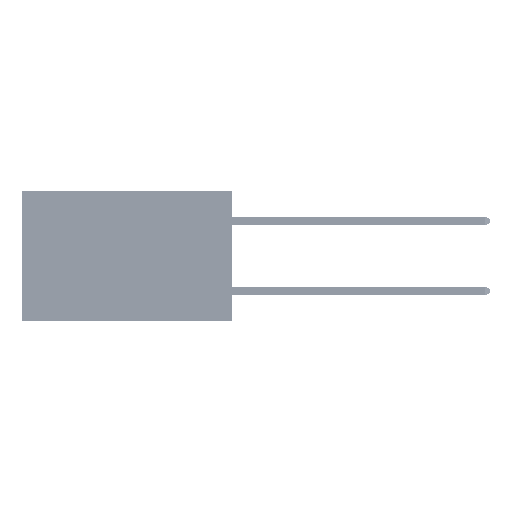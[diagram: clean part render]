
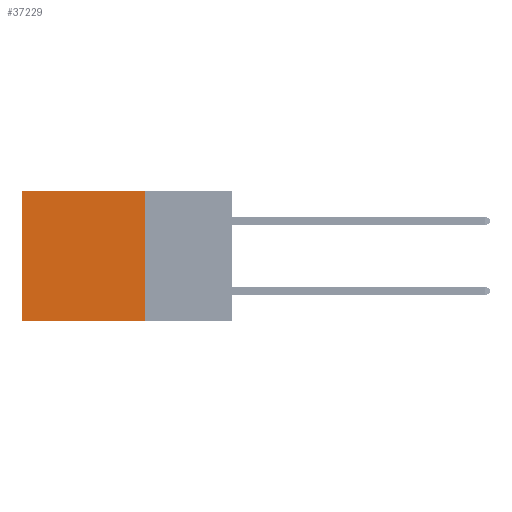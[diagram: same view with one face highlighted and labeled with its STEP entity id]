
A CAD part, left-side view. The second image highlights one B-rep face of the part: STEP entity #37229.
In plain terms, the highlighted planar face has unit normal (-1, 0, 0).
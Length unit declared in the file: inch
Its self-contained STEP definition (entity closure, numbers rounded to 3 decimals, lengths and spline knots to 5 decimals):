
#192 = CARTESIAN_POINT ( 'NONE',  ( 0.2875, 0.25, 0. ) ) ;
#3415 = VECTOR ( 'NONE', #33637, 39.37008 ) ;
#3467 = EDGE_CURVE ( 'NONE', #28301, #17805, #35521, .T. ) ;
#4042 = ORIENTED_EDGE ( 'NONE', *, *, #40278, .T. ) ;
#5532 = CARTESIAN_POINT ( 'NONE',  ( 0.2875, 0.25, -0.37 ) ) ;
#6696 = VERTEX_POINT ( 'NONE', #23124 ) ;
#11294 = VECTOR ( 'NONE', #22963, 39.37008 ) ;
#14636 = EDGE_CURVE ( 'NONE', #6696, #17805, #23315, .T. ) ;
#15011 = LINE ( 'NONE', #192, #49844 ) ;
#15630 = CARTESIAN_POINT ( 'NONE',  ( 0.2875, 0.25, 0. ) ) ;
#17805 = VERTEX_POINT ( 'NONE', #40143 ) ;
#22963 = DIRECTION ( 'NONE',  ( 0., 0., -1. ) ) ;
#23124 = CARTESIAN_POINT ( 'NONE',  ( 0.2875, 0.6, 0. ) ) ;
#23315 = LINE ( 'NONE', #30748, #11294 ) ;
#25441 = EDGE_LOOP ( 'NONE', ( #36223, #34992, #48789, #4042 ) ) ;
#28301 = VERTEX_POINT ( 'NONE', #50284 ) ;
#30748 = CARTESIAN_POINT ( 'NONE',  ( 0.2875, 0.6, 0. ) ) ;
#33637 = DIRECTION ( 'NONE',  ( 0., 1., 0. ) ) ;
#34992 = ORIENTED_EDGE ( 'NONE', *, *, #3467, .F. ) ;
#35521 = LINE ( 'NONE', #5532, #3415 ) ;
#36223 = ORIENTED_EDGE ( 'NONE', *, *, #14636, .T. ) ;
#36271 = DIRECTION ( 'NONE',  ( 0., 0., -1. ) ) ;
#37229 = ADVANCED_FACE ( 'NONE', ( #47916 ), #40158, .F. ) ;
#38785 = DIRECTION ( 'NONE',  ( 0., 1., 0. ) ) ;
#40143 = CARTESIAN_POINT ( 'NONE',  ( 0.2875, 0.6, -0.37 ) ) ;
#40158 = PLANE ( 'NONE',  #52076 ) ;
#40204 = DIRECTION ( 'NONE',  ( 0., 0., -1. ) ) ;
#40278 = EDGE_CURVE ( 'NONE', #47304, #6696, #47516, .T. ) ;
#42198 = CARTESIAN_POINT ( 'NONE',  ( 0.2875, 0.25, 0. ) ) ;
#44269 = CARTESIAN_POINT ( 'NONE',  ( 0.2875, 0.25, 0. ) ) ;
#47304 = VERTEX_POINT ( 'NONE', #15630 ) ;
#47516 = LINE ( 'NONE', #42198, #50661 ) ;
#47916 = FACE_OUTER_BOUND ( 'NONE', #25441, .T. ) ;
#48529 = DIRECTION ( 'NONE',  ( 1., 0., 0. ) ) ;
#48789 = ORIENTED_EDGE ( 'NONE', *, *, #51129, .F. ) ;
#49844 = VECTOR ( 'NONE', #40204, 39.37008 ) ;
#50284 = CARTESIAN_POINT ( 'NONE',  ( 0.2875, 0.25, -0.37 ) ) ;
#50661 = VECTOR ( 'NONE', #38785, 39.37008 ) ;
#51129 = EDGE_CURVE ( 'NONE', #47304, #28301, #15011, .T. ) ;
#52076 = AXIS2_PLACEMENT_3D ( 'NONE', #44269, #48529, #36271 ) ;
